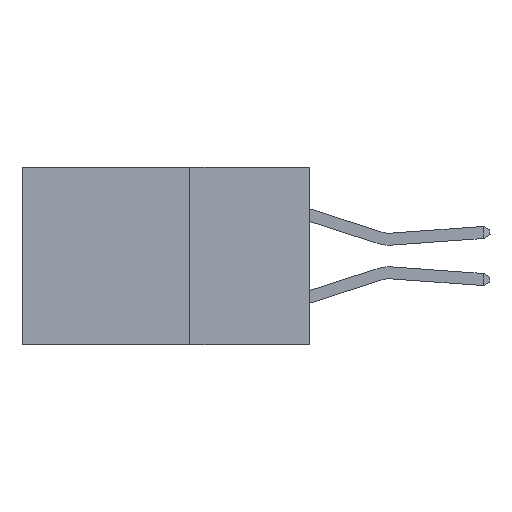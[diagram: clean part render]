
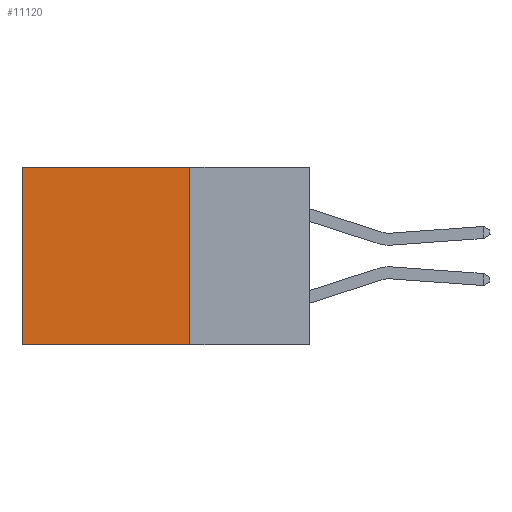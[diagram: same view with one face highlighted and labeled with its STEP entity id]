
A CAD part, left-side view. The second image highlights one B-rep face of the part: STEP entity #11120.
In plain terms, the highlighted planar face has unit normal (-1, 0, 0).
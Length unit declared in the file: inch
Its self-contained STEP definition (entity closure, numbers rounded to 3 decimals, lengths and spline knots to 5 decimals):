
#954 = VERTEX_POINT ( 'NONE', #2769 ) ;
#1256 = LINE ( 'NONE', #8229, #9696 ) ;
#1950 = DIRECTION ( 'NONE',  ( 0., 0., -1. ) ) ;
#2030 = EDGE_CURVE ( 'NONE', #13348, #4662, #14167, .T. ) ;
#2769 = CARTESIAN_POINT ( 'NONE',  ( 0.2615, 0.25, 0. ) ) ;
#2779 = EDGE_LOOP ( 'NONE', ( #12531, #5405, #7928, #4710 ) ) ;
#4198 = VECTOR ( 'NONE', #5695, 39.37008 ) ;
#4662 = VERTEX_POINT ( 'NONE', #18389 ) ;
#4710 = ORIENTED_EDGE ( 'NONE', *, *, #13194, .T. ) ;
#5405 = ORIENTED_EDGE ( 'NONE', *, *, #2030, .F. ) ;
#5516 = CARTESIAN_POINT ( 'NONE',  ( 0.2615, 0.25, -0.37 ) ) ;
#5682 = CARTESIAN_POINT ( 'NONE',  ( 0.2615, 0.25, -0.37 ) ) ;
#5695 = DIRECTION ( 'NONE',  ( 0., 1., 0. ) ) ;
#6029 = VECTOR ( 'NONE', #10842, 39.37008 ) ;
#6989 = VECTOR ( 'NONE', #11426, 39.37008 ) ;
#7270 = LINE ( 'NONE', #5682, #6989 ) ;
#7584 = FACE_OUTER_BOUND ( 'NONE', #2779, .T. ) ;
#7928 = ORIENTED_EDGE ( 'NONE', *, *, #11408, .F. ) ;
#8229 = CARTESIAN_POINT ( 'NONE',  ( 0.2615, 0.25, 0. ) ) ;
#8396 = CARTESIAN_POINT ( 'NONE',  ( 0.2615, 0.6, 0. ) ) ;
#8580 = VERTEX_POINT ( 'NONE', #8396 ) ;
#9093 = CARTESIAN_POINT ( 'NONE',  ( 0.2615, 0.25, -0.37 ) ) ;
#9334 = CARTESIAN_POINT ( 'NONE',  ( 0.2615, 0.6, -0.37 ) ) ;
#9696 = VECTOR ( 'NONE', #17049, 39.37008 ) ;
#9723 = EDGE_CURVE ( 'NONE', #8580, #4662, #11985, .T. ) ;
#10378 = CARTESIAN_POINT ( 'NONE',  ( 0.2615, 0.25, -0.37 ) ) ;
#10842 = DIRECTION ( 'NONE',  ( 0., 0., -1. ) ) ;
#11120 = ADVANCED_FACE ( 'NONE', ( #7584 ), #16222, .F. ) ;
#11408 = EDGE_CURVE ( 'NONE', #954, #13348, #7270, .T. ) ;
#11426 = DIRECTION ( 'NONE',  ( 0., 0., -1. ) ) ;
#11500 = AXIS2_PLACEMENT_3D ( 'NONE', #9093, #14828, #1950 ) ;
#11985 = LINE ( 'NONE', #9334, #6029 ) ;
#12531 = ORIENTED_EDGE ( 'NONE', *, *, #9723, .T. ) ;
#13194 = EDGE_CURVE ( 'NONE', #954, #8580, #1256, .T. ) ;
#13348 = VERTEX_POINT ( 'NONE', #10378 ) ;
#14167 = LINE ( 'NONE', #5516, #4198 ) ;
#14828 = DIRECTION ( 'NONE',  ( 1., 0., 0. ) ) ;
#16222 = PLANE ( 'NONE',  #11500 ) ;
#17049 = DIRECTION ( 'NONE',  ( 0., 1., 0. ) ) ;
#18389 = CARTESIAN_POINT ( 'NONE',  ( 0.2615, 0.6, -0.37 ) ) ;
